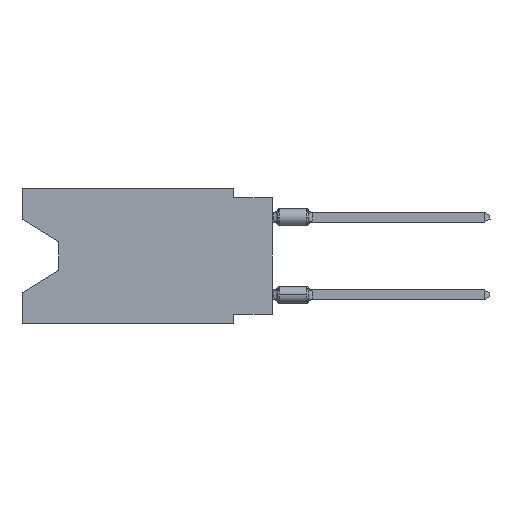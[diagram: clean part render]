
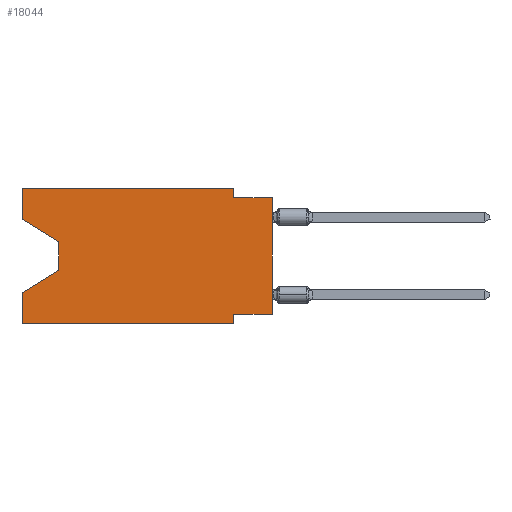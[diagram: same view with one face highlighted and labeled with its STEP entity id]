
A CAD part, left-side view. The second image highlights one B-rep face of the part: STEP entity #18044.
In plain terms, the highlighted planar face has unit normal (-1, 0, 0).
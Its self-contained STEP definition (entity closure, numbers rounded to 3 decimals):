
#314 = CARTESIAN_POINT ( 'NONE',  ( 0., 16.383, -8.89 ) ) ;
#704 = EDGE_CURVE ( 'NONE', #2085, #30028, #15262, .T. ) ;
#947 = CARTESIAN_POINT ( 'NONE',  ( 0., 16.383, 0. ) ) ;
#962 = VECTOR ( 'NONE', #7210, 1000. ) ;
#1134 = LINE ( 'NONE', #4762, #27200 ) ;
#1379 = VERTEX_POINT ( 'NONE', #13394 ) ;
#1385 = EDGE_CURVE ( 'NONE', #30199, #39193, #1134, .T. ) ;
#1813 = VECTOR ( 'NONE', #16133, 1000. ) ;
#2067 = LINE ( 'NONE', #13909, #30644 ) ;
#2085 = VERTEX_POINT ( 'NONE', #314 ) ;
#2260 = VECTOR ( 'NONE', #21905, 1000. ) ;
#2357 = AXIS2_PLACEMENT_3D ( 'NONE', #30239, #20981, #12505 ) ;
#2480 = CARTESIAN_POINT ( 'NONE',  ( 0., 16.383, 0. ) ) ;
#2921 = ORIENTED_EDGE ( 'NONE', *, *, #12361, .T. ) ;
#3149 = ORIENTED_EDGE ( 'NONE', *, *, #28727, .F. ) ;
#3184 = EDGE_LOOP ( 'NONE', ( #5165, #25257, #24205, #28926, #2921, #30350, #3149, #9246, #35096, #33825, #15472, #4383 ) ) ;
#4246 = CARTESIAN_POINT ( 'NONE',  ( 0., 2.54, 0. ) ) ;
#4259 = LINE ( 'NONE', #28794, #1813 ) ;
#4383 = ORIENTED_EDGE ( 'NONE', *, *, #35027, .F. ) ;
#4762 = CARTESIAN_POINT ( 'NONE',  ( 0., 0., -0.635 ) ) ;
#5165 = ORIENTED_EDGE ( 'NONE', *, *, #6388, .T. ) ;
#6388 = EDGE_CURVE ( 'NONE', #30368, #21773, #2067, .T. ) ;
#6429 = VERTEX_POINT ( 'NONE', #8093 ) ;
#6764 = VECTOR ( 'NONE', #38647, 1000. ) ;
#7210 = DIRECTION ( 'NONE',  ( 0., -1., 0. ) ) ;
#7775 = DIRECTION ( 'NONE',  ( 0., 0.855, -0.519 ) ) ;
#7848 = CARTESIAN_POINT ( 'NONE',  ( 0., 0., 0. ) ) ;
#7954 = LINE ( 'NONE', #23645, #35006 ) ;
#8093 = CARTESIAN_POINT ( 'NONE',  ( 0., 13.97, -5.385 ) ) ;
#8680 = DIRECTION ( 'NONE',  ( 0., -1., 0. ) ) ;
#9246 = ORIENTED_EDGE ( 'NONE', *, *, #16844, .T. ) ;
#10394 = DIRECTION ( 'NONE',  ( 0., -1., 0. ) ) ;
#11110 = VERTEX_POINT ( 'NONE', #35648 ) ;
#12116 = FACE_OUTER_BOUND ( 'NONE', #3184, .T. ) ;
#12361 = EDGE_CURVE ( 'NONE', #2085, #35646, #26790, .T. ) ;
#12505 = DIRECTION ( 'NONE',  ( 0., 0., -1. ) ) ;
#13073 = LINE ( 'NONE', #4246, #20409 ) ;
#13288 = CARTESIAN_POINT ( 'NONE',  ( 0., 2.54, -8.89 ) ) ;
#13394 = CARTESIAN_POINT ( 'NONE',  ( 0., 0., -8.255 ) ) ;
#13664 = DIRECTION ( 'NONE',  ( 0., 0., -1. ) ) ;
#13909 = CARTESIAN_POINT ( 'NONE',  ( 0., 16.383, -2.038 ) ) ;
#15262 = LINE ( 'NONE', #17904, #23925 ) ;
#15472 = ORIENTED_EDGE ( 'NONE', *, *, #18974, .F. ) ;
#16133 = DIRECTION ( 'NONE',  ( 0., 0., -1. ) ) ;
#16234 = CARTESIAN_POINT ( 'NONE',  ( 0., 0., -8.255 ) ) ;
#16239 = CARTESIAN_POINT ( 'NONE',  ( 0., 13.97, -3.505 ) ) ;
#16348 = CARTESIAN_POINT ( 'NONE',  ( 0., 2.54, 0. ) ) ;
#16640 = DIRECTION ( 'NONE',  ( 0., 1., 0. ) ) ;
#16844 = EDGE_CURVE ( 'NONE', #1379, #39193, #28987, .T. ) ;
#17312 = CARTESIAN_POINT ( 'NONE',  ( 0., 16.383, -6.852 ) ) ;
#17904 = CARTESIAN_POINT ( 'NONE',  ( 0., 16.383, 0. ) ) ;
#18044 = ADVANCED_FACE ( 'NONE', ( #12116 ), #21798, .F. ) ;
#18542 = VECTOR ( 'NONE', #8680, 1000. ) ;
#18616 = VECTOR ( 'NONE', #16640, 1000. ) ;
#18974 = EDGE_CURVE ( 'NONE', #27684, #33500, #34559, .T. ) ;
#18980 = CARTESIAN_POINT ( 'NONE',  ( 0., 13.97, -3.505 ) ) ;
#19048 = EDGE_CURVE ( 'NONE', #21773, #6429, #24901, .T. ) ;
#19622 = CARTESIAN_POINT ( 'NONE',  ( 0., 13.97, -5.385 ) ) ;
#20409 = VECTOR ( 'NONE', #13664, 1000. ) ;
#20423 = DIRECTION ( 'NONE',  ( 0., 0., 1. ) ) ;
#20981 = DIRECTION ( 'NONE',  ( 1., 0., 0. ) ) ;
#21010 = VECTOR ( 'NONE', #7775, 1000. ) ;
#21773 = VERTEX_POINT ( 'NONE', #18980 ) ;
#21798 = PLANE ( 'NONE',  #2357 ) ;
#21905 = DIRECTION ( 'NONE',  ( 0., 0., -1. ) ) ;
#22377 = EDGE_CURVE ( 'NONE', #33500, #30199, #13073, .T. ) ;
#22866 = LINE ( 'NONE', #16234, #18616 ) ;
#23645 = CARTESIAN_POINT ( 'NONE',  ( 0., 16.383, 0. ) ) ;
#23925 = VECTOR ( 'NONE', #27566, 1000. ) ;
#24205 = ORIENTED_EDGE ( 'NONE', *, *, #25872, .T. ) ;
#24901 = LINE ( 'NONE', #16239, #2260 ) ;
#25257 = ORIENTED_EDGE ( 'NONE', *, *, #19048, .T. ) ;
#25872 = EDGE_CURVE ( 'NONE', #6429, #30028, #32102, .T. ) ;
#26593 = CARTESIAN_POINT ( 'NONE',  ( 0., 16.383, -8.89 ) ) ;
#26790 = LINE ( 'NONE', #26593, #18542 ) ;
#26795 = EDGE_CURVE ( 'NONE', #11110, #35646, #4259, .T. ) ;
#27200 = VECTOR ( 'NONE', #10394, 1000. ) ;
#27566 = DIRECTION ( 'NONE',  ( 0., 0., 1. ) ) ;
#27684 = VERTEX_POINT ( 'NONE', #2480 ) ;
#28727 = EDGE_CURVE ( 'NONE', #1379, #11110, #22866, .T. ) ;
#28794 = CARTESIAN_POINT ( 'NONE',  ( 0., 2.54, -8.89 ) ) ;
#28926 = ORIENTED_EDGE ( 'NONE', *, *, #704, .F. ) ;
#28987 = LINE ( 'NONE', #7848, #6764 ) ;
#30028 = VERTEX_POINT ( 'NONE', #17312 ) ;
#30199 = VERTEX_POINT ( 'NONE', #39254 ) ;
#30239 = CARTESIAN_POINT ( 'NONE',  ( 0., 16.383, 0. ) ) ;
#30350 = ORIENTED_EDGE ( 'NONE', *, *, #26795, .F. ) ;
#30368 = VERTEX_POINT ( 'NONE', #38611 ) ;
#30644 = VECTOR ( 'NONE', #33217, 1000. ) ;
#32102 = LINE ( 'NONE', #19622, #21010 ) ;
#33217 = DIRECTION ( 'NONE',  ( 0., -0.855, -0.519 ) ) ;
#33500 = VERTEX_POINT ( 'NONE', #16348 ) ;
#33825 = ORIENTED_EDGE ( 'NONE', *, *, #22377, .F. ) ;
#34559 = LINE ( 'NONE', #947, #962 ) ;
#35006 = VECTOR ( 'NONE', #20423, 1000. ) ;
#35027 = EDGE_CURVE ( 'NONE', #30368, #27684, #7954, .T. ) ;
#35096 = ORIENTED_EDGE ( 'NONE', *, *, #1385, .F. ) ;
#35646 = VERTEX_POINT ( 'NONE', #13288 ) ;
#35648 = CARTESIAN_POINT ( 'NONE',  ( 0., 2.54, -8.255 ) ) ;
#35846 = CARTESIAN_POINT ( 'NONE',  ( 0., 0., -0.635 ) ) ;
#38611 = CARTESIAN_POINT ( 'NONE',  ( 0., 16.383, -2.038 ) ) ;
#38647 = DIRECTION ( 'NONE',  ( 0., 0., 1. ) ) ;
#39193 = VERTEX_POINT ( 'NONE', #35846 ) ;
#39254 = CARTESIAN_POINT ( 'NONE',  ( 0., 2.54, -0.635 ) ) ;
